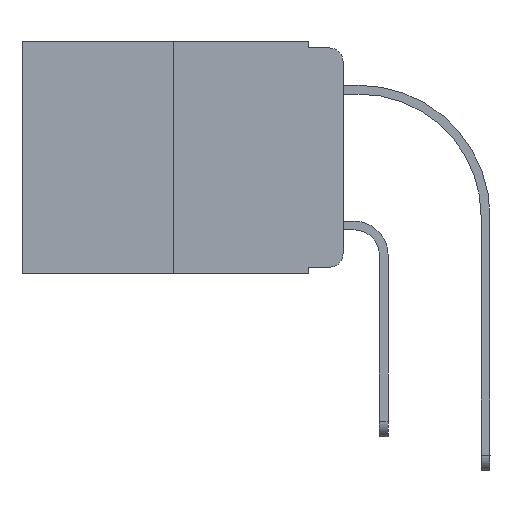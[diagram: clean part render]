
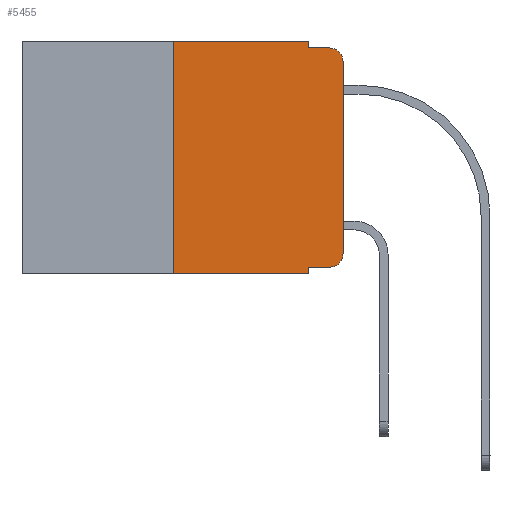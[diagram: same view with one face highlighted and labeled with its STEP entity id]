
A CAD part, left-side view. The second image highlights one B-rep face of the part: STEP entity #5455.
In plain terms, the highlighted planar face has unit normal (-1, 0, 0).
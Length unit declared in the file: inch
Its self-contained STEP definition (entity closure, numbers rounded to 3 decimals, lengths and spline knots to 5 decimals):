
#331 = CARTESIAN_POINT ( 'NONE',  ( 0., 0.25, 0. ) ) ;
#1166 = DIRECTION ( 'NONE',  ( 0., 0., -1. ) ) ;
#1544 = VERTEX_POINT ( 'NONE', #24993 ) ;
#1634 = LINE ( 'NONE', #18070, #24508 ) ;
#1867 = CARTESIAN_POINT ( 'NONE',  ( 0., 0.051, -0.333 ) ) ;
#1917 = EDGE_CURVE ( 'NONE', #22784, #5576, #2348, .T. ) ;
#2290 = DIRECTION ( 'NONE',  ( 0., -1., 0. ) ) ;
#2348 = LINE ( 'NONE', #14584, #12284 ) ;
#2405 = DIRECTION ( 'NONE',  ( -1., 0., 0. ) ) ;
#2831 = VERTEX_POINT ( 'NONE', #331 ) ;
#3128 = DIRECTION ( 'NONE',  ( 0., -1., 0. ) ) ;
#3132 = CARTESIAN_POINT ( 'NONE',  ( 0., 0.02, -0.01 ) ) ;
#3399 = CIRCLE ( 'NONE', #13296, 0.02 ) ;
#3698 = ORIENTED_EDGE ( 'NONE', *, *, #15941, .T. ) ;
#4644 = ORIENTED_EDGE ( 'NONE', *, *, #9122, .F. ) ;
#4773 = DIRECTION ( 'NONE',  ( 0., -1., 0. ) ) ;
#5455 = ADVANCED_FACE ( 'NONE', ( #16953 ), #8347, .F. ) ;
#5523 = EDGE_CURVE ( 'NONE', #2831, #1544, #20574, .T. ) ;
#5542 = LINE ( 'NONE', #13752, #15933 ) ;
#5576 = VERTEX_POINT ( 'NONE', #13435 ) ;
#7068 = ORIENTED_EDGE ( 'NONE', *, *, #15168, .F. ) ;
#7269 = VECTOR ( 'NONE', #20265, 39.37008 ) ;
#8103 = LINE ( 'NONE', #10128, #23691 ) ;
#8347 = PLANE ( 'NONE',  #11835 ) ;
#8916 = EDGE_CURVE ( 'NONE', #17347, #18358, #5542, .T. ) ;
#9122 = EDGE_CURVE ( 'NONE', #17347, #5576, #1634, .T. ) ;
#9256 = EDGE_LOOP ( 'NONE', ( #19173, #17497, #7068, #18396, #25448, #10446, #20533, #4644, #13600, #3698 ) ) ;
#9486 = AXIS2_PLACEMENT_3D ( 'NONE', #21626, #26036, #1166 ) ;
#10041 = DIRECTION ( 'NONE',  ( 0., -1., 0. ) ) ;
#10128 = CARTESIAN_POINT ( 'NONE',  ( 0., 0.25, 0. ) ) ;
#10331 = EDGE_CURVE ( 'NONE', #22784, #2831, #8103, .T. ) ;
#10446 = ORIENTED_EDGE ( 'NONE', *, *, #10331, .F. ) ;
#11835 = AXIS2_PLACEMENT_3D ( 'NONE', #16825, #14507, #24853 ) ;
#12051 = LINE ( 'NONE', #15810, #12449 ) ;
#12284 = VECTOR ( 'NONE', #4773, 39.37008 ) ;
#12313 = LINE ( 'NONE', #18513, #23150 ) ;
#12449 = VECTOR ( 'NONE', #10041, 39.37008 ) ;
#13296 = AXIS2_PLACEMENT_3D ( 'NONE', #24607, #2405, #22858 ) ;
#13435 = CARTESIAN_POINT ( 'NONE',  ( 0., 0.051, -0.343 ) ) ;
#13600 = ORIENTED_EDGE ( 'NONE', *, *, #8916, .T. ) ;
#13752 = CARTESIAN_POINT ( 'NONE',  ( 0., 0.051, -0.333 ) ) ;
#14022 = DIRECTION ( 'NONE',  ( 0., 0., 1. ) ) ;
#14095 = VERTEX_POINT ( 'NONE', #3132 ) ;
#14204 = CIRCLE ( 'NONE', #9486, 0.02 ) ;
#14507 = DIRECTION ( 'NONE',  ( 1., 0., 0. ) ) ;
#14584 = CARTESIAN_POINT ( 'NONE',  ( 0., 0.473, -0.343 ) ) ;
#15130 = EDGE_CURVE ( 'NONE', #1544, #25630, #19866, .T. ) ;
#15168 = EDGE_CURVE ( 'NONE', #25630, #14095, #12051, .T. ) ;
#15627 = CARTESIAN_POINT ( 'NONE',  ( 0., 0.25, -0.343 ) ) ;
#15810 = CARTESIAN_POINT ( 'NONE',  ( 0., 0.051, -0.01 ) ) ;
#15933 = VECTOR ( 'NONE', #3128, 39.37008 ) ;
#15941 = EDGE_CURVE ( 'NONE', #18358, #24869, #14204, .T. ) ;
#16825 = CARTESIAN_POINT ( 'NONE',  ( 0., 0.473, 0. ) ) ;
#16953 = FACE_OUTER_BOUND ( 'NONE', #9256, .T. ) ;
#17347 = VERTEX_POINT ( 'NONE', #1867 ) ;
#17497 = ORIENTED_EDGE ( 'NONE', *, *, #19855, .T. ) ;
#17831 = EDGE_CURVE ( 'NONE', #24869, #20789, #12313, .T. ) ;
#18070 = CARTESIAN_POINT ( 'NONE',  ( 0., 0.051, 0. ) ) ;
#18358 = VERTEX_POINT ( 'NONE', #19371 ) ;
#18396 = ORIENTED_EDGE ( 'NONE', *, *, #15130, .F. ) ;
#18513 = CARTESIAN_POINT ( 'NONE',  ( 0., 0., 0. ) ) ;
#19168 = CARTESIAN_POINT ( 'NONE',  ( 0., 0., -0.313 ) ) ;
#19173 = ORIENTED_EDGE ( 'NONE', *, *, #17831, .T. ) ;
#19371 = CARTESIAN_POINT ( 'NONE',  ( 0., 0.02, -0.333 ) ) ;
#19855 = EDGE_CURVE ( 'NONE', #20789, #14095, #3399, .T. ) ;
#19866 = LINE ( 'NONE', #24142, #7269 ) ;
#20265 = DIRECTION ( 'NONE',  ( 0., 0., -1. ) ) ;
#20533 = ORIENTED_EDGE ( 'NONE', *, *, #1917, .T. ) ;
#20574 = LINE ( 'NONE', #23097, #21247 ) ;
#20657 = DIRECTION ( 'NONE',  ( 0., 0., 1. ) ) ;
#20789 = VERTEX_POINT ( 'NONE', #21299 ) ;
#21247 = VECTOR ( 'NONE', #2290, 39.37008 ) ;
#21299 = CARTESIAN_POINT ( 'NONE',  ( 0., 0., -0.03 ) ) ;
#21626 = CARTESIAN_POINT ( 'NONE',  ( 0., 0.02, -0.313 ) ) ;
#22592 = CARTESIAN_POINT ( 'NONE',  ( 0., 0.051, -0.01 ) ) ;
#22784 = VERTEX_POINT ( 'NONE', #15627 ) ;
#22858 = DIRECTION ( 'NONE',  ( 0., 0., -1. ) ) ;
#23097 = CARTESIAN_POINT ( 'NONE',  ( 0., 0.473, 0. ) ) ;
#23150 = VECTOR ( 'NONE', #20657, 39.37008 ) ;
#23691 = VECTOR ( 'NONE', #14022, 39.37008 ) ;
#24142 = CARTESIAN_POINT ( 'NONE',  ( 0., 0.051, 0. ) ) ;
#24227 = DIRECTION ( 'NONE',  ( 0., 0., -1. ) ) ;
#24508 = VECTOR ( 'NONE', #24227, 39.37008 ) ;
#24607 = CARTESIAN_POINT ( 'NONE',  ( 0., 0.02, -0.03 ) ) ;
#24853 = DIRECTION ( 'NONE',  ( 0., 0., -1. ) ) ;
#24869 = VERTEX_POINT ( 'NONE', #19168 ) ;
#24993 = CARTESIAN_POINT ( 'NONE',  ( 0., 0.051, 0. ) ) ;
#25448 = ORIENTED_EDGE ( 'NONE', *, *, #5523, .F. ) ;
#25630 = VERTEX_POINT ( 'NONE', #22592 ) ;
#26036 = DIRECTION ( 'NONE',  ( -1., 0., 0. ) ) ;
